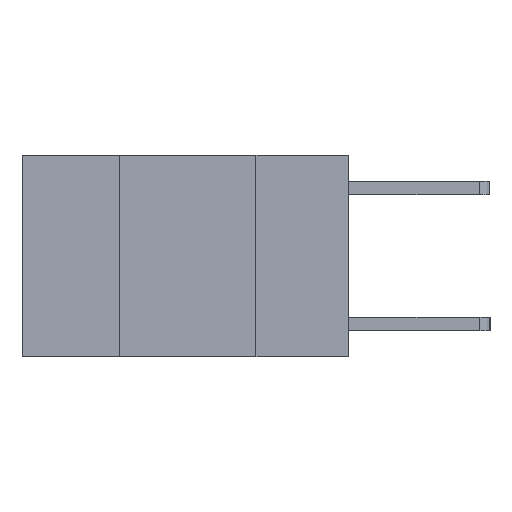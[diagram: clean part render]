
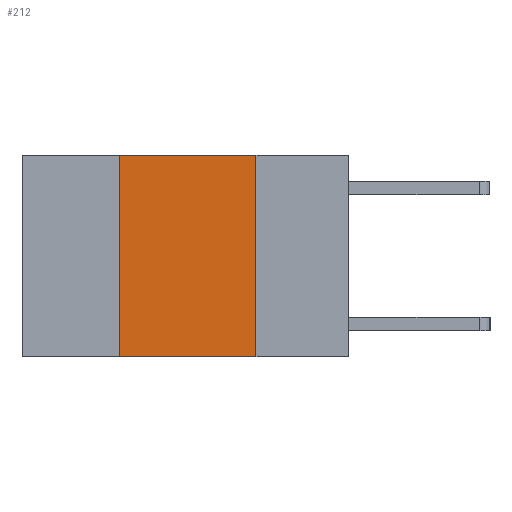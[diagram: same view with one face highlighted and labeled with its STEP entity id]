
A CAD part, left-side view. The second image highlights one B-rep face of the part: STEP entity #212.
In plain terms, the highlighted planar face has unit normal (-1, 0, 0).
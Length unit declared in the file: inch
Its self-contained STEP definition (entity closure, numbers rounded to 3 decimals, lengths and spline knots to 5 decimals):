
#212 = ADVANCED_FACE ( 'NONE', ( #6080 ), #3719, .F. ) ;
#691 = DIRECTION ( 'NONE',  ( 0., 0., 1. ) ) ;
#735 = CARTESIAN_POINT ( 'NONE',  ( 0., 0.42, 0. ) ) ;
#757 = VECTOR ( 'NONE', #7295, 39.37008 ) ;
#1251 = ORIENTED_EDGE ( 'NONE', *, *, #4405, .F. ) ;
#1824 = CARTESIAN_POINT ( 'NONE',  ( 0., 0.6, 0. ) ) ;
#1982 = CARTESIAN_POINT ( 'NONE',  ( 0., 0.6, 0. ) ) ;
#1986 = VERTEX_POINT ( 'NONE', #2451 ) ;
#2002 = VERTEX_POINT ( 'NONE', #2356 ) ;
#2356 = CARTESIAN_POINT ( 'NONE',  ( 0., 0.42, -0.37 ) ) ;
#2391 = EDGE_CURVE ( 'NONE', #6627, #7975, #6171, .T. ) ;
#2451 = CARTESIAN_POINT ( 'NONE',  ( 0., 0.42, 0. ) ) ;
#3302 = EDGE_CURVE ( 'NONE', #2002, #7975, #5467, .T. ) ;
#3719 = PLANE ( 'NONE',  #7122 ) ;
#3977 = ORIENTED_EDGE ( 'NONE', *, *, #7951, .F. ) ;
#4282 = EDGE_LOOP ( 'NONE', ( #6086, #3977, #1251, #8597 ) ) ;
#4302 = CARTESIAN_POINT ( 'NONE',  ( 0., 0.17, 0. ) ) ;
#4405 = EDGE_CURVE ( 'NONE', #2002, #1986, #5858, .T. ) ;
#4443 = VECTOR ( 'NONE', #8091, 39.37008 ) ;
#4573 = LINE ( 'NONE', #1982, #757 ) ;
#5057 = DIRECTION ( 'NONE',  ( 0., -1., 0. ) ) ;
#5129 = CARTESIAN_POINT ( 'NONE',  ( 0., 0.6, -0.37 ) ) ;
#5467 = LINE ( 'NONE', #5129, #7003 ) ;
#5858 = LINE ( 'NONE', #735, #7597 ) ;
#5994 = DIRECTION ( 'NONE',  ( 0., 0., -1. ) ) ;
#6080 = FACE_OUTER_BOUND ( 'NONE', #4282, .T. ) ;
#6086 = ORIENTED_EDGE ( 'NONE', *, *, #2391, .F. ) ;
#6171 = LINE ( 'NONE', #8155, #4443 ) ;
#6554 = DIRECTION ( 'NONE',  ( 1., 0., 0. ) ) ;
#6627 = VERTEX_POINT ( 'NONE', #4302 ) ;
#7003 = VECTOR ( 'NONE', #5057, 39.37008 ) ;
#7122 = AXIS2_PLACEMENT_3D ( 'NONE', #1824, #6554, #5994 ) ;
#7295 = DIRECTION ( 'NONE',  ( 0., -1., 0. ) ) ;
#7597 = VECTOR ( 'NONE', #691, 39.37008 ) ;
#7951 = EDGE_CURVE ( 'NONE', #1986, #6627, #4573, .T. ) ;
#7975 = VERTEX_POINT ( 'NONE', #8600 ) ;
#8091 = DIRECTION ( 'NONE',  ( 0., 0., -1. ) ) ;
#8155 = CARTESIAN_POINT ( 'NONE',  ( 0., 0.17, 0. ) ) ;
#8597 = ORIENTED_EDGE ( 'NONE', *, *, #3302, .T. ) ;
#8600 = CARTESIAN_POINT ( 'NONE',  ( 0., 0.17, -0.37 ) ) ;
